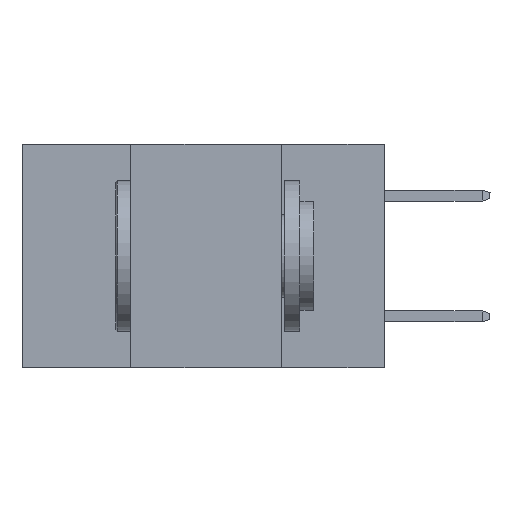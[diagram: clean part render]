
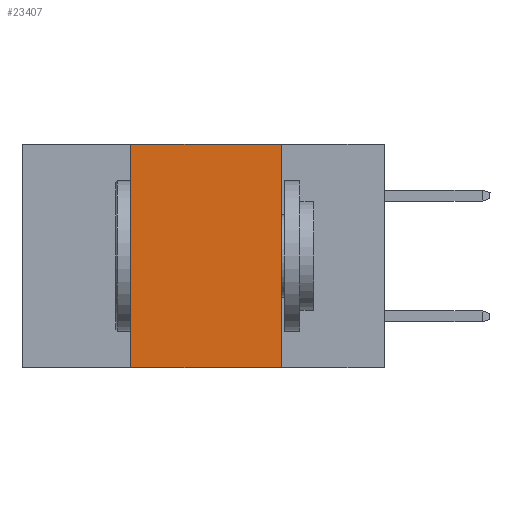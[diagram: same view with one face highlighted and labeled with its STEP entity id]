
A CAD part, left-side view. The second image highlights one B-rep face of the part: STEP entity #23407.
In plain terms, the highlighted planar face has unit normal (-1, 0, 0).
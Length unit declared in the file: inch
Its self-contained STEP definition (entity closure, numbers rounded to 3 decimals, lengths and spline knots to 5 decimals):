
#35 = LINE ( 'NONE', #11181, #12764 ) ;
#1265 = CARTESIAN_POINT ( 'NONE',  ( 0., 0.6, -0.37 ) ) ;
#1980 = VECTOR ( 'NONE', #3687, 39.37008 ) ;
#3687 = DIRECTION ( 'NONE',  ( 0., -1., 0. ) ) ;
#4265 = CARTESIAN_POINT ( 'NONE',  ( 0., 0.42, -0.37 ) ) ;
#4646 = ORIENTED_EDGE ( 'NONE', *, *, #10414, .F. ) ;
#4672 = CARTESIAN_POINT ( 'NONE',  ( 0., 0.6, 0. ) ) ;
#4712 = DIRECTION ( 'NONE',  ( 0., 0., 1. ) ) ;
#6000 = VERTEX_POINT ( 'NONE', #28970 ) ;
#6141 = ORIENTED_EDGE ( 'NONE', *, *, #13971, .T. ) ;
#6561 = FACE_OUTER_BOUND ( 'NONE', #11533, .T. ) ;
#7166 = LINE ( 'NONE', #11801, #13188 ) ;
#9459 = ORIENTED_EDGE ( 'NONE', *, *, #25131, .F. ) ;
#10414 = EDGE_CURVE ( 'NONE', #17331, #6000, #27855, .T. ) ;
#11181 = CARTESIAN_POINT ( 'NONE',  ( 0., 0.17, 0. ) ) ;
#11533 = EDGE_LOOP ( 'NONE', ( #9459, #4646, #17375, #6141 ) ) ;
#11801 = CARTESIAN_POINT ( 'NONE',  ( 0., 0.42, 0. ) ) ;
#12764 = VECTOR ( 'NONE', #27776, 39.37008 ) ;
#13188 = VECTOR ( 'NONE', #4712, 39.37008 ) ;
#13971 = EDGE_CURVE ( 'NONE', #19958, #27384, #14690, .T. ) ;
#14135 = DIRECTION ( 'NONE',  ( 0., -1., 0. ) ) ;
#14271 = DIRECTION ( 'NONE',  ( 0., 0., -1. ) ) ;
#14690 = LINE ( 'NONE', #1265, #1980 ) ;
#17228 = EDGE_CURVE ( 'NONE', #19958, #17331, #7166, .T. ) ;
#17331 = VERTEX_POINT ( 'NONE', #21704 ) ;
#17375 = ORIENTED_EDGE ( 'NONE', *, *, #17228, .F. ) ;
#19958 = VERTEX_POINT ( 'NONE', #4265 ) ;
#21396 = CARTESIAN_POINT ( 'NONE',  ( 0., 0.17, -0.37 ) ) ;
#21704 = CARTESIAN_POINT ( 'NONE',  ( 0., 0.42, 0. ) ) ;
#23407 = ADVANCED_FACE ( 'NONE', ( #6561 ), #23735, .F. ) ;
#23710 = AXIS2_PLACEMENT_3D ( 'NONE', #30781, #28488, #14271 ) ;
#23735 = PLANE ( 'NONE',  #23710 ) ;
#25131 = EDGE_CURVE ( 'NONE', #6000, #27384, #35, .T. ) ;
#26389 = VECTOR ( 'NONE', #14135, 39.37008 ) ;
#27384 = VERTEX_POINT ( 'NONE', #21396 ) ;
#27776 = DIRECTION ( 'NONE',  ( 0., 0., -1. ) ) ;
#27855 = LINE ( 'NONE', #4672, #26389 ) ;
#28488 = DIRECTION ( 'NONE',  ( 1., 0., 0. ) ) ;
#28970 = CARTESIAN_POINT ( 'NONE',  ( 0., 0.17, 0. ) ) ;
#30781 = CARTESIAN_POINT ( 'NONE',  ( 0., 0.6, 0. ) ) ;
